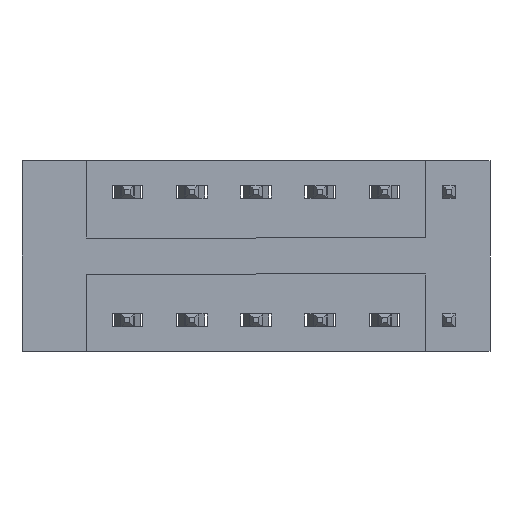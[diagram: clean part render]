
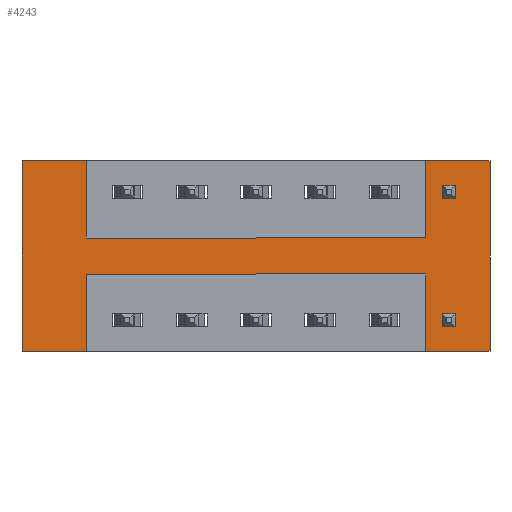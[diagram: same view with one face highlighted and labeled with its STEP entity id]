
A CAD part, front view. The second image highlights one B-rep face of the part: STEP entity #4243.
In plain terms, the highlighted planar face has unit normal (0, -1, 0).
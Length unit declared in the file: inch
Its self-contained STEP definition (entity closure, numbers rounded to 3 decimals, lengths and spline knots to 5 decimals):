
#90 = VERTEX_POINT ( 'NONE', #2594 ) ;
#102 = ORIENTED_EDGE ( 'NONE', *, *, #3910, .F. ) ;
#131 = FACE_OUTER_BOUND ( 'NONE', #5229, .T. ) ;
#164 = VECTOR ( 'NONE', #8009, 39.37008 ) ;
#249 = VERTEX_POINT ( 'NONE', #7098 ) ;
#298 = EDGE_CURVE ( 'NONE', #90, #2017, #5850, .T. ) ;
#471 = VERTEX_POINT ( 'NONE', #8067 ) ;
#619 = PLANE ( 'NONE',  #1066 ) ;
#749 = CARTESIAN_POINT ( 'NONE',  ( 0., 0., -0.37 ) ) ;
#799 = VECTOR ( 'NONE', #2691, 39.37008 ) ;
#854 = CARTESIAN_POINT ( 'NONE',  ( 1.0475, 0., -0.37 ) ) ;
#918 = ORIENTED_EDGE ( 'NONE', *, *, #6012, .F. ) ;
#952 = ORIENTED_EDGE ( 'NONE', *, *, #5106, .F. ) ;
#1000 = DIRECTION ( 'NONE',  ( 0., 0., 1. ) ) ;
#1066 = AXIS2_PLACEMENT_3D ( 'NONE', #749, #6869, #1312 ) ;
#1077 = CARTESIAN_POINT ( 'NONE',  ( 1.0475, 0., -0.22 ) ) ;
#1105 = DIRECTION ( 'NONE',  ( -1., 0., 0. ) ) ;
#1312 = DIRECTION ( 'NONE',  ( 0., 0., -1. ) ) ;
#1345 = LINE ( 'NONE', #3943, #1428 ) ;
#1417 = ORIENTED_EDGE ( 'NONE', *, *, #4296, .F. ) ;
#1426 = CARTESIAN_POINT ( 'NONE',  ( 1.1725, 0., 0. ) ) ;
#1428 = VECTOR ( 'NONE', #3986, 39.37008 ) ;
#1644 = LINE ( 'NONE', #6078, #6235 ) ;
#1855 = CARTESIAN_POINT ( 'NONE',  ( 0.3875, 0., -0.37 ) ) ;
#1856 = ORIENTED_EDGE ( 'NONE', *, *, #5384, .F. ) ;
#1932 = LINE ( 'NONE', #3678, #164 ) ;
#2017 = VERTEX_POINT ( 'NONE', #4122 ) ;
#2059 = LINE ( 'NONE', #6294, #3529 ) ;
#2138 = ORIENTED_EDGE ( 'NONE', *, *, #7543, .F. ) ;
#2195 = DIRECTION ( 'NONE',  ( 0., 0., 1. ) ) ;
#2204 = DIRECTION ( 'NONE',  ( 0., 0., 1. ) ) ;
#2398 = VERTEX_POINT ( 'NONE', #854 ) ;
#2422 = LINE ( 'NONE', #1855, #4586 ) ;
#2518 = EDGE_CURVE ( 'NONE', #90, #471, #4919, .T. ) ;
#2594 = CARTESIAN_POINT ( 'NONE',  ( 0.2625, 0., 0. ) ) ;
#2596 = VECTOR ( 'NONE', #2195, 39.37008 ) ;
#2630 = CARTESIAN_POINT ( 'NONE',  ( 1.0475, 0., 0. ) ) ;
#2691 = DIRECTION ( 'NONE',  ( 0., 0., -1. ) ) ;
#2734 = VERTEX_POINT ( 'NONE', #4713 ) ;
#2815 = LINE ( 'NONE', #4108, #6279 ) ;
#2880 = VECTOR ( 'NONE', #7242, 39.37008 ) ;
#2911 = ORIENTED_EDGE ( 'NONE', *, *, #6656, .F. ) ;
#2941 = ORIENTED_EDGE ( 'NONE', *, *, #298, .F. ) ;
#3025 = ORIENTED_EDGE ( 'NONE', *, *, #7208, .F. ) ;
#3080 = CARTESIAN_POINT ( 'NONE',  ( 0.2625, 0., 0. ) ) ;
#3306 = VERTEX_POINT ( 'NONE', #2630 ) ;
#3341 = CARTESIAN_POINT ( 'NONE',  ( 0.3875, 0., 0. ) ) ;
#3364 = VECTOR ( 'NONE', #7270, 39.37008 ) ;
#3404 = DIRECTION ( 'NONE',  ( 1., 0., 0. ) ) ;
#3465 = CARTESIAN_POINT ( 'NONE',  ( 0.3875, 0., -0.22 ) ) ;
#3529 = VECTOR ( 'NONE', #3964, 39.37008 ) ;
#3654 = VECTOR ( 'NONE', #1105, 39.37008 ) ;
#3678 = CARTESIAN_POINT ( 'NONE',  ( 0., 0., -0.37 ) ) ;
#3910 = EDGE_CURVE ( 'NONE', #2734, #4173, #2059, .T. ) ;
#3943 = CARTESIAN_POINT ( 'NONE',  ( 0., 0., 0. ) ) ;
#3964 = DIRECTION ( 'NONE',  ( 1., 0., 0. ) ) ;
#3986 = DIRECTION ( 'NONE',  ( 1., 0., 0. ) ) ;
#4010 = CARTESIAN_POINT ( 'NONE',  ( 0., 0., 0. ) ) ;
#4039 = VERTEX_POINT ( 'NONE', #6830 ) ;
#4108 = CARTESIAN_POINT ( 'NONE',  ( 1.0475, 0., 0. ) ) ;
#4122 = CARTESIAN_POINT ( 'NONE',  ( 0.3875, 0., 0. ) ) ;
#4173 = VERTEX_POINT ( 'NONE', #6737 ) ;
#4243 = ADVANCED_FACE ( 'NONE', ( #131 ), #619, .T. ) ;
#4296 = EDGE_CURVE ( 'NONE', #2398, #5007, #4996, .T. ) ;
#4356 = DIRECTION ( 'NONE',  ( 0., 0., -1. ) ) ;
#4586 = VECTOR ( 'NONE', #4356, 39.37008 ) ;
#4684 = EDGE_CURVE ( 'NONE', #3306, #5560, #1345, .T. ) ;
#4713 = CARTESIAN_POINT ( 'NONE',  ( 0.3875, 0., -0.15 ) ) ;
#4919 = LINE ( 'NONE', #3080, #3364 ) ;
#4990 = EDGE_CURVE ( 'NONE', #249, #5560, #1644, .T. ) ;
#4996 = LINE ( 'NONE', #7467, #2596 ) ;
#5007 = VERTEX_POINT ( 'NONE', #1077 ) ;
#5106 = EDGE_CURVE ( 'NONE', #7457, #471, #6782, .T. ) ;
#5229 = EDGE_LOOP ( 'NONE', ( #6881, #7843, #2138, #102, #1856, #2941, #7988, #952, #918, #2911, #1417, #3025 ) ) ;
#5384 = EDGE_CURVE ( 'NONE', #2017, #2734, #6998, .T. ) ;
#5560 = VERTEX_POINT ( 'NONE', #1426 ) ;
#5850 = LINE ( 'NONE', #4010, #8008 ) ;
#5940 = CARTESIAN_POINT ( 'NONE',  ( 0.3875, 0., -0.37 ) ) ;
#6012 = EDGE_CURVE ( 'NONE', #4039, #7457, #2422, .T. ) ;
#6068 = LINE ( 'NONE', #3465, #2880 ) ;
#6078 = CARTESIAN_POINT ( 'NONE',  ( 1.1725, 0., 0. ) ) ;
#6235 = VECTOR ( 'NONE', #1000, 39.37008 ) ;
#6279 = VECTOR ( 'NONE', #2204, 39.37008 ) ;
#6294 = CARTESIAN_POINT ( 'NONE',  ( 0.3875, 0., -0.15 ) ) ;
#6656 = EDGE_CURVE ( 'NONE', #5007, #4039, #6068, .T. ) ;
#6737 = CARTESIAN_POINT ( 'NONE',  ( 1.0475, 0., -0.15 ) ) ;
#6782 = LINE ( 'NONE', #7455, #3654 ) ;
#6830 = CARTESIAN_POINT ( 'NONE',  ( 0.3875, 0., -0.22 ) ) ;
#6869 = DIRECTION ( 'NONE',  ( 0., -1., 0. ) ) ;
#6881 = ORIENTED_EDGE ( 'NONE', *, *, #4990, .T. ) ;
#6998 = LINE ( 'NONE', #3341, #799 ) ;
#7098 = CARTESIAN_POINT ( 'NONE',  ( 1.1725, 0., -0.37 ) ) ;
#7208 = EDGE_CURVE ( 'NONE', #249, #2398, #1932, .T. ) ;
#7242 = DIRECTION ( 'NONE',  ( -1., 0., 0. ) ) ;
#7270 = DIRECTION ( 'NONE',  ( 0., 0., -1. ) ) ;
#7455 = CARTESIAN_POINT ( 'NONE',  ( 0., 0., -0.37 ) ) ;
#7457 = VERTEX_POINT ( 'NONE', #5940 ) ;
#7467 = CARTESIAN_POINT ( 'NONE',  ( 1.0475, 0., -0.37 ) ) ;
#7543 = EDGE_CURVE ( 'NONE', #4173, #3306, #2815, .T. ) ;
#7843 = ORIENTED_EDGE ( 'NONE', *, *, #4684, .F. ) ;
#7988 = ORIENTED_EDGE ( 'NONE', *, *, #2518, .T. ) ;
#8008 = VECTOR ( 'NONE', #3404, 39.37008 ) ;
#8009 = DIRECTION ( 'NONE',  ( -1., 0., 0. ) ) ;
#8067 = CARTESIAN_POINT ( 'NONE',  ( 0.2625, 0., -0.37 ) ) ;
